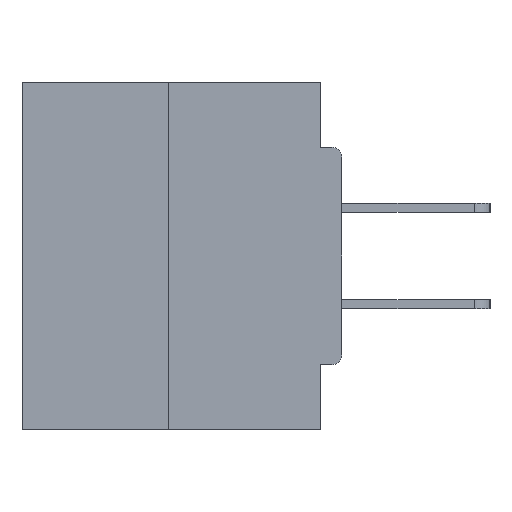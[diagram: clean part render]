
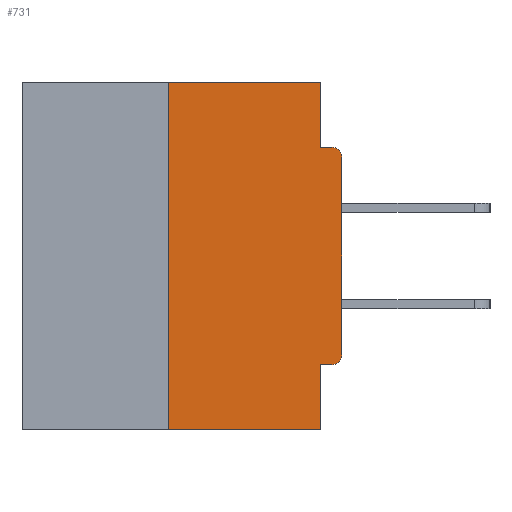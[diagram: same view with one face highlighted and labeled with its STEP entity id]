
A CAD part, left-side view. The second image highlights one B-rep face of the part: STEP entity #731.
In plain terms, the highlighted planar face has unit normal (-1, 0, 0).
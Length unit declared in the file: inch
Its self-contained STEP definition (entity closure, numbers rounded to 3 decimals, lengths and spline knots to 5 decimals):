
#731 = ADVANCED_FACE ( 'NONE', ( #31011 ), #30415, .F. ) ;
#737 = EDGE_LOOP ( 'NONE', ( #34848, #25029, #26320, #3198, #21632, #38628, #27761, #16514, #2942, #36390 ) ) ;
#1116 = EDGE_CURVE ( 'NONE', #26366, #31525, #17268, .T. ) ;
#2322 = EDGE_CURVE ( 'NONE', #5452, #26366, #3160, .T. ) ;
#2625 = VECTOR ( 'NONE', #8987, 39.37008 ) ;
#2942 = ORIENTED_EDGE ( 'NONE', *, *, #36443, .F. ) ;
#3160 = LINE ( 'NONE', #27844, #17631 ) ;
#3198 = ORIENTED_EDGE ( 'NONE', *, *, #28717, .F. ) ;
#3625 = LINE ( 'NONE', #16360, #17769 ) ;
#4895 = LINE ( 'NONE', #29538, #35633 ) ;
#5452 = VERTEX_POINT ( 'NONE', #6164 ) ;
#5582 = AXIS2_PLACEMENT_3D ( 'NONE', #37301, #6177, #12622 ) ;
#6164 = CARTESIAN_POINT ( 'NONE',  ( 0., 0.25, -0.5 ) ) ;
#6177 = DIRECTION ( 'NONE',  ( 1., 0., 0. ) ) ;
#6319 = CARTESIAN_POINT ( 'NONE',  ( 0., 0.46, -0.5 ) ) ;
#6620 = CARTESIAN_POINT ( 'NONE',  ( 0., 0.015, -0.3915 ) ) ;
#6847 = CARTESIAN_POINT ( 'NONE',  ( 0., 0.25, 0. ) ) ;
#7388 = VERTEX_POINT ( 'NONE', #30625 ) ;
#8987 = DIRECTION ( 'NONE',  ( 0., -1., 0. ) ) ;
#9347 = AXIS2_PLACEMENT_3D ( 'NONE', #13340, #34982, #38445 ) ;
#9435 = LINE ( 'NONE', #23683, #19311 ) ;
#9747 = VERTEX_POINT ( 'NONE', #12698 ) ;
#10341 = EDGE_CURVE ( 'NONE', #7388, #29000, #33882, .T. ) ;
#10645 = CARTESIAN_POINT ( 'NONE',  ( 0., 0.015, -0.0935 ) ) ;
#12196 = LINE ( 'NONE', #18266, #2625 ) ;
#12622 = DIRECTION ( 'NONE',  ( 0., 0., -1. ) ) ;
#12631 = CARTESIAN_POINT ( 'NONE',  ( 0., 0.031, -0.4065 ) ) ;
#12698 = CARTESIAN_POINT ( 'NONE',  ( 0., 0.031, -0.5 ) ) ;
#13340 = CARTESIAN_POINT ( 'NONE',  ( 0., 0.015, -0.1085 ) ) ;
#13587 = EDGE_CURVE ( 'NONE', #31525, #37510, #3625, .T. ) ;
#14168 = DIRECTION ( 'NONE',  ( 0., 1., 0. ) ) ;
#15670 = VERTEX_POINT ( 'NONE', #27679 ) ;
#15755 = VECTOR ( 'NONE', #20425, 39.37008 ) ;
#16360 = CARTESIAN_POINT ( 'NONE',  ( 0., 0.031, 0. ) ) ;
#16514 = ORIENTED_EDGE ( 'NONE', *, *, #10341, .T. ) ;
#16529 = DIRECTION ( 'NONE',  ( 0., 0., -1. ) ) ;
#16563 = VECTOR ( 'NONE', #27938, 39.37008 ) ;
#17207 = CARTESIAN_POINT ( 'NONE',  ( 0., 0.031, 0. ) ) ;
#17268 = LINE ( 'NONE', #35680, #34550 ) ;
#17631 = VECTOR ( 'NONE', #21184, 39.37008 ) ;
#17769 = VECTOR ( 'NONE', #25061, 39.37008 ) ;
#18266 = CARTESIAN_POINT ( 'NONE',  ( 0., 0., -0.0935 ) ) ;
#18818 = LINE ( 'NONE', #6319, #16563 ) ;
#19311 = VECTOR ( 'NONE', #35814, 39.37008 ) ;
#20425 = DIRECTION ( 'NONE',  ( 0., 0., 1. ) ) ;
#20930 = CARTESIAN_POINT ( 'NONE',  ( 0., 0.031, -0.0935 ) ) ;
#21184 = DIRECTION ( 'NONE',  ( 0., 0., 1. ) ) ;
#21632 = ORIENTED_EDGE ( 'NONE', *, *, #32849, .F. ) ;
#23322 = EDGE_CURVE ( 'NONE', #31166, #15670, #23419, .T. ) ;
#23419 = CIRCLE ( 'NONE', #25324, 0.015 ) ;
#23683 = CARTESIAN_POINT ( 'NONE',  ( 0., 0.031, -0.5 ) ) ;
#24096 = EDGE_CURVE ( 'NONE', #5452, #9747, #18818, .T. ) ;
#24871 = VERTEX_POINT ( 'NONE', #12631 ) ;
#25029 = ORIENTED_EDGE ( 'NONE', *, *, #2322, .F. ) ;
#25061 = DIRECTION ( 'NONE',  ( 0., 0., -1. ) ) ;
#25324 = AXIS2_PLACEMENT_3D ( 'NONE', #6620, #37549, #16529 ) ;
#26320 = ORIENTED_EDGE ( 'NONE', *, *, #24096, .T. ) ;
#26366 = VERTEX_POINT ( 'NONE', #6847 ) ;
#27679 = CARTESIAN_POINT ( 'NONE',  ( 0., 0., -0.3915 ) ) ;
#27761 = ORIENTED_EDGE ( 'NONE', *, *, #35457, .T. ) ;
#27844 = CARTESIAN_POINT ( 'NONE',  ( 0., 0.25, 0. ) ) ;
#27938 = DIRECTION ( 'NONE',  ( 0., -1., 0. ) ) ;
#28717 = EDGE_CURVE ( 'NONE', #24871, #9747, #9435, .T. ) ;
#29000 = VERTEX_POINT ( 'NONE', #10645 ) ;
#29538 = CARTESIAN_POINT ( 'NONE',  ( 0., 0., -0.4065 ) ) ;
#29579 = CARTESIAN_POINT ( 'NONE',  ( 0., 0.015, -0.4065 ) ) ;
#30415 = PLANE ( 'NONE',  #5582 ) ;
#30625 = CARTESIAN_POINT ( 'NONE',  ( 0., 0., -0.1085 ) ) ;
#31011 = FACE_OUTER_BOUND ( 'NONE', #737, .T. ) ;
#31166 = VERTEX_POINT ( 'NONE', #29579 ) ;
#31525 = VERTEX_POINT ( 'NONE', #17207 ) ;
#32849 = EDGE_CURVE ( 'NONE', #31166, #24871, #4895, .T. ) ;
#33882 = CIRCLE ( 'NONE', #9347, 0.015 ) ;
#34550 = VECTOR ( 'NONE', #39721, 39.37008 ) ;
#34848 = ORIENTED_EDGE ( 'NONE', *, *, #1116, .F. ) ;
#34982 = DIRECTION ( 'NONE',  ( -1., 0., 0. ) ) ;
#35457 = EDGE_CURVE ( 'NONE', #15670, #7388, #36181, .T. ) ;
#35633 = VECTOR ( 'NONE', #14168, 39.37008 ) ;
#35680 = CARTESIAN_POINT ( 'NONE',  ( 0., 0.46, 0. ) ) ;
#35803 = CARTESIAN_POINT ( 'NONE',  ( 0., 0., 0. ) ) ;
#35814 = DIRECTION ( 'NONE',  ( 0., 0., -1. ) ) ;
#36181 = LINE ( 'NONE', #35803, #15755 ) ;
#36390 = ORIENTED_EDGE ( 'NONE', *, *, #13587, .F. ) ;
#36443 = EDGE_CURVE ( 'NONE', #37510, #29000, #12196, .T. ) ;
#37301 = CARTESIAN_POINT ( 'NONE',  ( 0., 0.46, 0. ) ) ;
#37510 = VERTEX_POINT ( 'NONE', #20930 ) ;
#37549 = DIRECTION ( 'NONE',  ( -1., 0., 0. ) ) ;
#38445 = DIRECTION ( 'NONE',  ( 0., 0., -1. ) ) ;
#38628 = ORIENTED_EDGE ( 'NONE', *, *, #23322, .T. ) ;
#39721 = DIRECTION ( 'NONE',  ( 0., -1., 0. ) ) ;
